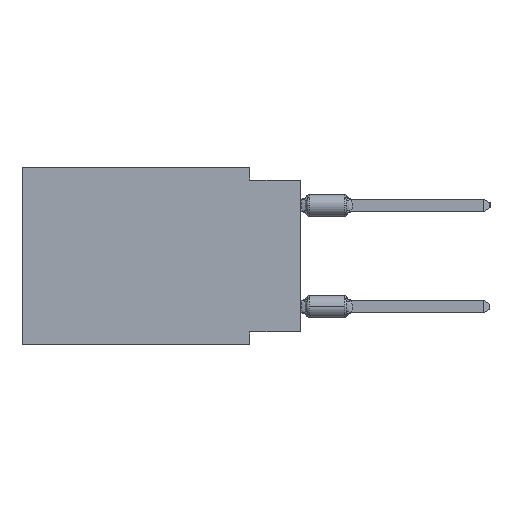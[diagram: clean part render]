
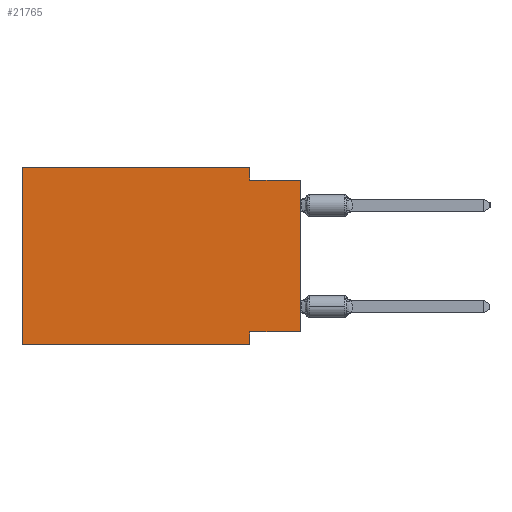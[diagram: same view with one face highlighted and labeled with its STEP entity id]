
A CAD part, left-side view. The second image highlights one B-rep face of the part: STEP entity #21765.
In plain terms, the highlighted planar face has unit normal (-1, 0, 0).
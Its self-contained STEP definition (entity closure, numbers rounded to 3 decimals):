
#379 = ORIENTED_EDGE ( 'NONE', *, *, #4692, .F. ) ;
#1267 = DIRECTION ( 'NONE',  ( 0., 0., -1. ) ) ;
#1361 = EDGE_CURVE ( 'NONE', #4980, #19239, #7271, .T. ) ;
#1863 = CARTESIAN_POINT ( 'NONE',  ( 0., 13.97, 0. ) ) ;
#2313 = CARTESIAN_POINT ( 'NONE',  ( 0., 13.97, -8.89 ) ) ;
#2633 = DIRECTION ( 'NONE',  ( 0., -1., 0. ) ) ;
#3382 = EDGE_CURVE ( 'NONE', #4980, #6906, #27360, .T. ) ;
#3571 = CARTESIAN_POINT ( 'NONE',  ( 0., 13.97, 0. ) ) ;
#4692 = EDGE_CURVE ( 'NONE', #21776, #25940, #21714, .T. ) ;
#4790 = ORIENTED_EDGE ( 'NONE', *, *, #8730, .F. ) ;
#4958 = CARTESIAN_POINT ( 'NONE',  ( 0., 2.54, 0. ) ) ;
#4980 = VERTEX_POINT ( 'NONE', #26672 ) ;
#5024 = VECTOR ( 'NONE', #15776, 1000. ) ;
#5732 = DIRECTION ( 'NONE',  ( 0., 0., -1. ) ) ;
#6049 = ORIENTED_EDGE ( 'NONE', *, *, #7400, .T. ) ;
#6130 = VERTEX_POINT ( 'NONE', #13563 ) ;
#6902 = ORIENTED_EDGE ( 'NONE', *, *, #9887, .F. ) ;
#6906 = VERTEX_POINT ( 'NONE', #23338 ) ;
#7271 = LINE ( 'NONE', #21671, #29648 ) ;
#7400 = EDGE_CURVE ( 'NONE', #21776, #24172, #26124, .T. ) ;
#7755 = CARTESIAN_POINT ( 'NONE',  ( 0., 13.97, 0. ) ) ;
#8041 = VERTEX_POINT ( 'NONE', #10847 ) ;
#8175 = CARTESIAN_POINT ( 'NONE',  ( 0., 2.54, -8.89 ) ) ;
#8626 = CARTESIAN_POINT ( 'NONE',  ( 0., 0., -0.635 ) ) ;
#8730 = EDGE_CURVE ( 'NONE', #8041, #6906, #10985, .T. ) ;
#9512 = DIRECTION ( 'NONE',  ( 0., 0., -1. ) ) ;
#9584 = VECTOR ( 'NONE', #2633, 1000. ) ;
#9887 = EDGE_CURVE ( 'NONE', #6130, #8041, #21398, .T. ) ;
#10414 = CARTESIAN_POINT ( 'NONE',  ( 0., 13.97, -8.89 ) ) ;
#10773 = DIRECTION ( 'NONE',  ( 0., 0., 1. ) ) ;
#10847 = CARTESIAN_POINT ( 'NONE',  ( 0., 2.54, -0.635 ) ) ;
#10985 = LINE ( 'NONE', #8626, #15057 ) ;
#12706 = LINE ( 'NONE', #8175, #13469 ) ;
#13469 = VECTOR ( 'NONE', #1267, 1000. ) ;
#13563 = CARTESIAN_POINT ( 'NONE',  ( 0., 2.54, 0. ) ) ;
#13659 = EDGE_CURVE ( 'NONE', #19239, #24172, #12706, .T. ) ;
#14187 = EDGE_CURVE ( 'NONE', #25940, #6130, #30034, .T. ) ;
#14665 = CARTESIAN_POINT ( 'NONE',  ( 0., 2.54, -8.89 ) ) ;
#15057 = VECTOR ( 'NONE', #23048, 1000. ) ;
#15776 = DIRECTION ( 'NONE',  ( 0., -1., 0. ) ) ;
#16814 = DIRECTION ( 'NONE',  ( 0., 1., 0. ) ) ;
#19239 = VERTEX_POINT ( 'NONE', #27732 ) ;
#19662 = FACE_OUTER_BOUND ( 'NONE', #26924, .T. ) ;
#19753 = ORIENTED_EDGE ( 'NONE', *, *, #13659, .F. ) ;
#19811 = DIRECTION ( 'NONE',  ( 1., 0., 0. ) ) ;
#19973 = CARTESIAN_POINT ( 'NONE',  ( 0., 13.97, 0. ) ) ;
#21104 = VECTOR ( 'NONE', #27015, 1000. ) ;
#21398 = LINE ( 'NONE', #4958, #26119 ) ;
#21648 = AXIS2_PLACEMENT_3D ( 'NONE', #7755, #19811, #5732 ) ;
#21671 = CARTESIAN_POINT ( 'NONE',  ( 0., 0., -8.255 ) ) ;
#21714 = LINE ( 'NONE', #19973, #21104 ) ;
#21765 = ADVANCED_FACE ( 'NONE', ( #19662 ), #29209, .F. ) ;
#21776 = VERTEX_POINT ( 'NONE', #10414 ) ;
#23048 = DIRECTION ( 'NONE',  ( 0., -1., 0. ) ) ;
#23338 = CARTESIAN_POINT ( 'NONE',  ( 0., 0., -0.635 ) ) ;
#24172 = VERTEX_POINT ( 'NONE', #14665 ) ;
#24516 = ORIENTED_EDGE ( 'NONE', *, *, #3382, .T. ) ;
#25940 = VERTEX_POINT ( 'NONE', #3571 ) ;
#26119 = VECTOR ( 'NONE', #9512, 1000. ) ;
#26124 = LINE ( 'NONE', #2313, #9584 ) ;
#26672 = CARTESIAN_POINT ( 'NONE',  ( 0., 0., -8.255 ) ) ;
#26826 = ORIENTED_EDGE ( 'NONE', *, *, #1361, .F. ) ;
#26924 = EDGE_LOOP ( 'NONE', ( #24516, #4790, #6902, #29465, #379, #6049, #19753, #26826 ) ) ;
#27015 = DIRECTION ( 'NONE',  ( 0., 0., 1. ) ) ;
#27360 = LINE ( 'NONE', #29574, #28049 ) ;
#27732 = CARTESIAN_POINT ( 'NONE',  ( 0., 2.54, -8.255 ) ) ;
#28049 = VECTOR ( 'NONE', #10773, 1000. ) ;
#29209 = PLANE ( 'NONE',  #21648 ) ;
#29465 = ORIENTED_EDGE ( 'NONE', *, *, #14187, .F. ) ;
#29574 = CARTESIAN_POINT ( 'NONE',  ( 0., 0., 0. ) ) ;
#29648 = VECTOR ( 'NONE', #16814, 1000. ) ;
#30034 = LINE ( 'NONE', #1863, #5024 ) ;
